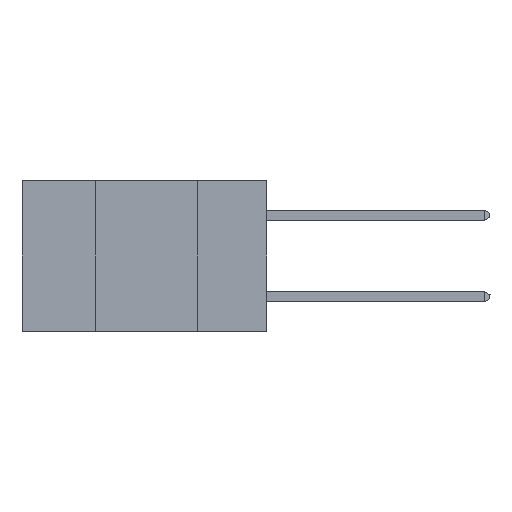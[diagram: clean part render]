
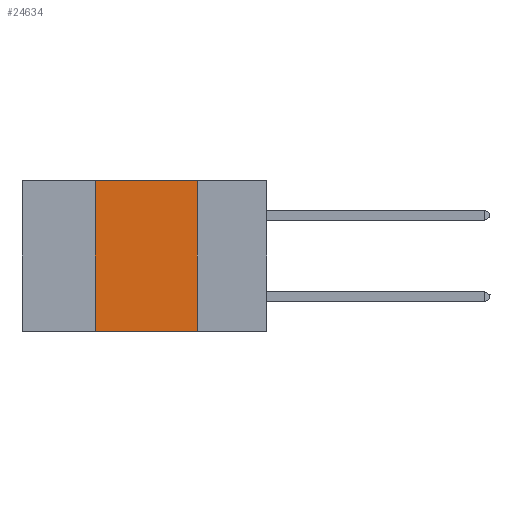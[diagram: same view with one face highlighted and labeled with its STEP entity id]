
A CAD part, left-side view. The second image highlights one B-rep face of the part: STEP entity #24634.
In plain terms, the highlighted planar face has unit normal (-1, 0, 0).
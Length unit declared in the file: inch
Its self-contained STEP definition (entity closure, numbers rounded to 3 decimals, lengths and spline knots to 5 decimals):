
#486 = VERTEX_POINT ( 'NONE', #5726 ) ;
#2832 = EDGE_CURVE ( 'NONE', #486, #24823, #8378, .T. ) ;
#3154 = LINE ( 'NONE', #14056, #3818 ) ;
#3254 = CARTESIAN_POINT ( 'NONE',  ( 0., 0.6, 0. ) ) ;
#3818 = VECTOR ( 'NONE', #10045, 39.37008 ) ;
#4169 = ORIENTED_EDGE ( 'NONE', *, *, #8638, .F. ) ;
#4236 = ORIENTED_EDGE ( 'NONE', *, *, #13787, .T. ) ;
#4725 = EDGE_CURVE ( 'NONE', #24823, #19064, #3154, .T. ) ;
#5242 = CARTESIAN_POINT ( 'NONE',  ( 0., 0.17, -0.37 ) ) ;
#5396 = DIRECTION ( 'NONE',  ( 0., -1., 0. ) ) ;
#5696 = LINE ( 'NONE', #12965, #17495 ) ;
#5726 = CARTESIAN_POINT ( 'NONE',  ( 0., 0.42, 0. ) ) ;
#7317 = EDGE_LOOP ( 'NONE', ( #16897, #13957, #4169, #4236 ) ) ;
#8378 = LINE ( 'NONE', #20246, #21490 ) ;
#8638 = EDGE_CURVE ( 'NONE', #16221, #486, #5696, .T. ) ;
#8953 = DIRECTION ( 'NONE',  ( 0., -1., 0. ) ) ;
#9017 = LINE ( 'NONE', #13162, #19744 ) ;
#9867 = DIRECTION ( 'NONE',  ( 0., 0., -1. ) ) ;
#9911 = FACE_OUTER_BOUND ( 'NONE', #7317, .T. ) ;
#10045 = DIRECTION ( 'NONE',  ( 0., 0., -1. ) ) ;
#12965 = CARTESIAN_POINT ( 'NONE',  ( 0., 0.42, 0. ) ) ;
#13162 = CARTESIAN_POINT ( 'NONE',  ( 0., 0.6, -0.37 ) ) ;
#13787 = EDGE_CURVE ( 'NONE', #16221, #19064, #9017, .T. ) ;
#13957 = ORIENTED_EDGE ( 'NONE', *, *, #2832, .F. ) ;
#14056 = CARTESIAN_POINT ( 'NONE',  ( 0., 0.17, 0. ) ) ;
#15031 = DIRECTION ( 'NONE',  ( 0., 0., 1. ) ) ;
#16166 = PLANE ( 'NONE',  #16817 ) ;
#16221 = VERTEX_POINT ( 'NONE', #24335 ) ;
#16817 = AXIS2_PLACEMENT_3D ( 'NONE', #3254, #20570, #9867 ) ;
#16897 = ORIENTED_EDGE ( 'NONE', *, *, #4725, .F. ) ;
#17495 = VECTOR ( 'NONE', #15031, 39.37008 ) ;
#19064 = VERTEX_POINT ( 'NONE', #5242 ) ;
#19744 = VECTOR ( 'NONE', #8953, 39.37008 ) ;
#20246 = CARTESIAN_POINT ( 'NONE',  ( 0., 0.6, 0. ) ) ;
#20570 = DIRECTION ( 'NONE',  ( 1., 0., 0. ) ) ;
#21490 = VECTOR ( 'NONE', #5396, 39.37008 ) ;
#24335 = CARTESIAN_POINT ( 'NONE',  ( 0., 0.42, -0.37 ) ) ;
#24634 = ADVANCED_FACE ( 'NONE', ( #9911 ), #16166, .F. ) ;
#24823 = VERTEX_POINT ( 'NONE', #26412 ) ;
#26412 = CARTESIAN_POINT ( 'NONE',  ( 0., 0.17, 0. ) ) ;
